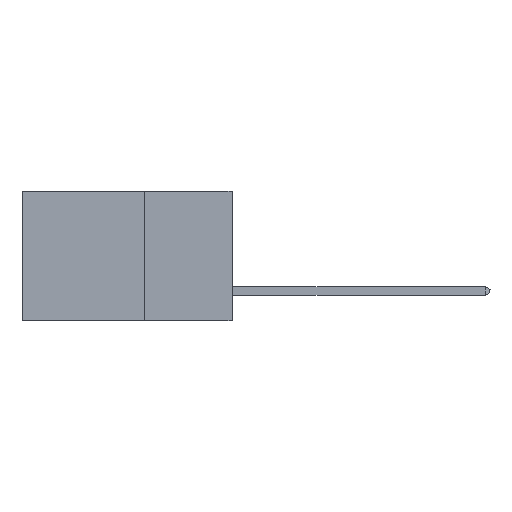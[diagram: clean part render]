
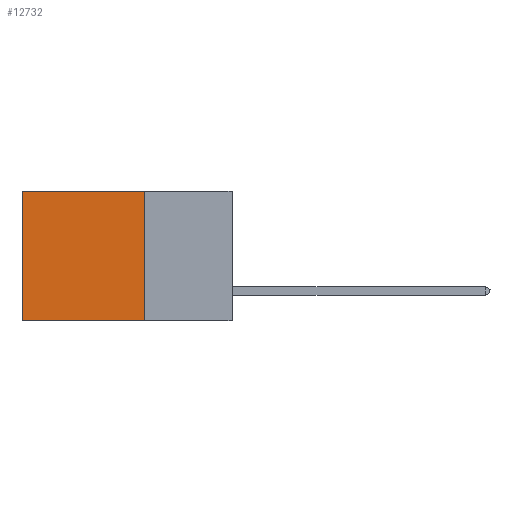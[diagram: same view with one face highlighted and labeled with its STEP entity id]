
A CAD part, left-side view. The second image highlights one B-rep face of the part: STEP entity #12732.
In plain terms, the highlighted planar face has unit normal (-1, 0, 0).
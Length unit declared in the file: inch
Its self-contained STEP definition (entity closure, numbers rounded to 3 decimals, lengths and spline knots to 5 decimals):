
#603 = VERTEX_POINT ( 'NONE', #6065 ) ;
#960 = CARTESIAN_POINT ( 'NONE',  ( 0.2875, 0.25, 0. ) ) ;
#1017 = CARTESIAN_POINT ( 'NONE',  ( 0.2875, 0.25, 0. ) ) ;
#1259 = LINE ( 'NONE', #11827, #9744 ) ;
#2463 = LINE ( 'NONE', #960, #4831 ) ;
#2649 = DIRECTION ( 'NONE',  ( 0., 0., -1. ) ) ;
#3037 = VERTEX_POINT ( 'NONE', #8982 ) ;
#3078 = FACE_OUTER_BOUND ( 'NONE', #14236, .T. ) ;
#3246 = ORIENTED_EDGE ( 'NONE', *, *, #7220, .F. ) ;
#3857 = EDGE_CURVE ( 'NONE', #12073, #603, #2463, .T. ) ;
#4004 = AXIS2_PLACEMENT_3D ( 'NONE', #13148, #13036, #10856 ) ;
#4126 = VECTOR ( 'NONE', #14938, 39.37008 ) ;
#4387 = LINE ( 'NONE', #9897, #9656 ) ;
#4831 = VECTOR ( 'NONE', #7923, 39.37008 ) ;
#4856 = CARTESIAN_POINT ( 'NONE',  ( 0.2875, 0.25, 0. ) ) ;
#4867 = LINE ( 'NONE', #1017, #4126 ) ;
#4964 = VERTEX_POINT ( 'NONE', #7254 ) ;
#6065 = CARTESIAN_POINT ( 'NONE',  ( 0.2875, 0.6, 0. ) ) ;
#6426 = DIRECTION ( 'NONE',  ( 0., 1., 0. ) ) ;
#7220 = EDGE_CURVE ( 'NONE', #12073, #4964, #4867, .T. ) ;
#7254 = CARTESIAN_POINT ( 'NONE',  ( 0.2875, 0.25, -0.37 ) ) ;
#7300 = ORIENTED_EDGE ( 'NONE', *, *, #13776, .T. ) ;
#7923 = DIRECTION ( 'NONE',  ( 0., 1., 0. ) ) ;
#8766 = ORIENTED_EDGE ( 'NONE', *, *, #10797, .F. ) ;
#8982 = CARTESIAN_POINT ( 'NONE',  ( 0.2875, 0.6, -0.37 ) ) ;
#9656 = VECTOR ( 'NONE', #6426, 39.37008 ) ;
#9744 = VECTOR ( 'NONE', #2649, 39.37008 ) ;
#9897 = CARTESIAN_POINT ( 'NONE',  ( 0.2875, 0.25, -0.37 ) ) ;
#10797 = EDGE_CURVE ( 'NONE', #4964, #3037, #4387, .T. ) ;
#10856 = DIRECTION ( 'NONE',  ( 0., 0., -1. ) ) ;
#11827 = CARTESIAN_POINT ( 'NONE',  ( 0.2875, 0.6, 0. ) ) ;
#11873 = PLANE ( 'NONE',  #4004 ) ;
#12073 = VERTEX_POINT ( 'NONE', #4856 ) ;
#12276 = ORIENTED_EDGE ( 'NONE', *, *, #3857, .T. ) ;
#12732 = ADVANCED_FACE ( 'NONE', ( #3078 ), #11873, .F. ) ;
#13036 = DIRECTION ( 'NONE',  ( 1., 0., 0. ) ) ;
#13148 = CARTESIAN_POINT ( 'NONE',  ( 0.2875, 0.25, 0. ) ) ;
#13776 = EDGE_CURVE ( 'NONE', #603, #3037, #1259, .T. ) ;
#14236 = EDGE_LOOP ( 'NONE', ( #7300, #8766, #3246, #12276 ) ) ;
#14938 = DIRECTION ( 'NONE',  ( 0., 0., -1. ) ) ;
